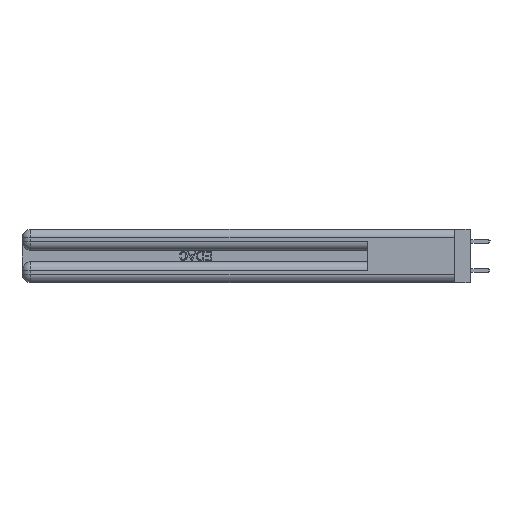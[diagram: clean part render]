
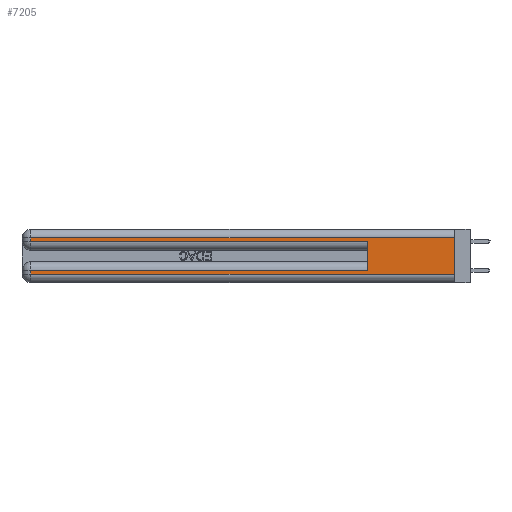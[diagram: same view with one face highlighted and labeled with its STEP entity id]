
A CAD part, left-side view. The second image highlights one B-rep face of the part: STEP entity #7205.
In plain terms, the highlighted planar face has unit normal (-1, 0, 0).
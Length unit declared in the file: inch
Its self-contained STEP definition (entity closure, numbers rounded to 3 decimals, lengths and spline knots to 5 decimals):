
#960 = EDGE_CURVE ( 'NONE', #34014, #14285, #3994, .T. ) ;
#1255 = CARTESIAN_POINT ( 'NONE',  ( 0., 0., 0.31 ) ) ;
#2277 = VECTOR ( 'NONE', #10742, 39.37008 ) ;
#3436 = CARTESIAN_POINT ( 'NONE',  ( 0., 0.6, 0.085 ) ) ;
#3994 = LINE ( 'NONE', #7187, #33371 ) ;
#4987 = ORIENTED_EDGE ( 'NONE', *, *, #38704, .T. ) ;
#5442 = LINE ( 'NONE', #36831, #28363 ) ;
#5456 = ORIENTED_EDGE ( 'NONE', *, *, #41916, .T. ) ;
#7187 = CARTESIAN_POINT ( 'NONE',  ( 0., 0.6, 0.145 ) ) ;
#7205 = ADVANCED_FACE ( 'NONE', ( #30709 ), #28962, .F. ) ;
#8068 = EDGE_CURVE ( 'NONE', #26083, #13559, #33846, .T. ) ;
#8346 = LINE ( 'NONE', #22822, #39291 ) ;
#10742 = DIRECTION ( 'NONE',  ( 0., 1., 0. ) ) ;
#10837 = VERTEX_POINT ( 'NONE', #41813 ) ;
#10854 = VECTOR ( 'NONE', #26650, 39.37008 ) ;
#11271 = CARTESIAN_POINT ( 'NONE',  ( 0., 0., 0.31 ) ) ;
#11644 = VECTOR ( 'NONE', #25696, 39.37008 ) ;
#11915 = LINE ( 'NONE', #27533, #2277 ) ;
#12110 = DIRECTION ( 'NONE',  ( 0., 0., -1. ) ) ;
#12236 = ORIENTED_EDGE ( 'NONE', *, *, #42745, .T. ) ;
#12563 = DIRECTION ( 'NONE',  ( 1., 0., 0. ) ) ;
#12837 = DIRECTION ( 'NONE',  ( 0., 0., -1. ) ) ;
#12926 = EDGE_LOOP ( 'NONE', ( #39824, #5456, #31135, #44123, #21703, #4987, #12236, #15629 ) ) ;
#13356 = VECTOR ( 'NONE', #18758, 39.37008 ) ;
#13559 = VERTEX_POINT ( 'NONE', #26681 ) ;
#14285 = VERTEX_POINT ( 'NONE', #33269 ) ;
#15629 = ORIENTED_EDGE ( 'NONE', *, *, #28323, .T. ) ;
#18758 = DIRECTION ( 'NONE',  ( 0., -1., 0. ) ) ;
#18905 = CARTESIAN_POINT ( 'NONE',  ( 0., 0., 0.06 ) ) ;
#20135 = EDGE_CURVE ( 'NONE', #41696, #10837, #23077, .T. ) ;
#20142 = EDGE_CURVE ( 'NONE', #10837, #14285, #5442, .T. ) ;
#20270 = CARTESIAN_POINT ( 'NONE',  ( 0., 2.94, 0.37 ) ) ;
#21246 = CARTESIAN_POINT ( 'NONE',  ( 0., 0., 0.37 ) ) ;
#21703 = ORIENTED_EDGE ( 'NONE', *, *, #960, .F. ) ;
#22822 = CARTESIAN_POINT ( 'NONE',  ( 0., 2.94, 0.37 ) ) ;
#23077 = LINE ( 'NONE', #20270, #10854 ) ;
#25696 = DIRECTION ( 'NONE',  ( 0., 1., 0. ) ) ;
#26083 = VERTEX_POINT ( 'NONE', #11271 ) ;
#26650 = DIRECTION ( 'NONE',  ( 0., 0., -1. ) ) ;
#26681 = CARTESIAN_POINT ( 'NONE',  ( 0., 0., 0.06 ) ) ;
#27533 = CARTESIAN_POINT ( 'NONE',  ( 0., 0., 0.085 ) ) ;
#28323 = EDGE_CURVE ( 'NONE', #43450, #13559, #40567, .T. ) ;
#28363 = VECTOR ( 'NONE', #40254, 39.37008 ) ;
#28826 = DIRECTION ( 'NONE',  ( 0., 0., -1. ) ) ;
#28962 = PLANE ( 'NONE',  #32299 ) ;
#29760 = CARTESIAN_POINT ( 'NONE',  ( 0., 2.94, 0.31 ) ) ;
#30709 = FACE_OUTER_BOUND ( 'NONE', #12926, .T. ) ;
#31049 = DIRECTION ( 'NONE',  ( 0., 0., 1. ) ) ;
#31135 = ORIENTED_EDGE ( 'NONE', *, *, #20135, .T. ) ;
#31692 = VECTOR ( 'NONE', #28826, 39.37008 ) ;
#32299 = AXIS2_PLACEMENT_3D ( 'NONE', #32560, #12563, #12110 ) ;
#32560 = CARTESIAN_POINT ( 'NONE',  ( 0., 0., 0.37 ) ) ;
#33269 = CARTESIAN_POINT ( 'NONE',  ( 0., 0.6, 0.285 ) ) ;
#33371 = VECTOR ( 'NONE', #31049, 39.37008 ) ;
#33846 = LINE ( 'NONE', #21246, #31692 ) ;
#34014 = VERTEX_POINT ( 'NONE', #3436 ) ;
#36831 = CARTESIAN_POINT ( 'NONE',  ( 0., 0., 0.285 ) ) ;
#38704 = EDGE_CURVE ( 'NONE', #34014, #42170, #11915, .T. ) ;
#38861 = LINE ( 'NONE', #1255, #11644 ) ;
#39291 = VECTOR ( 'NONE', #12837, 39.37008 ) ;
#39824 = ORIENTED_EDGE ( 'NONE', *, *, #8068, .F. ) ;
#39988 = CARTESIAN_POINT ( 'NONE',  ( 0., 2.94, 0.06 ) ) ;
#40174 = CARTESIAN_POINT ( 'NONE',  ( 0., 2.94, 0.085 ) ) ;
#40254 = DIRECTION ( 'NONE',  ( 0., -1., 0. ) ) ;
#40567 = LINE ( 'NONE', #18905, #13356 ) ;
#41696 = VERTEX_POINT ( 'NONE', #29760 ) ;
#41813 = CARTESIAN_POINT ( 'NONE',  ( 0., 2.94, 0.285 ) ) ;
#41916 = EDGE_CURVE ( 'NONE', #26083, #41696, #38861, .T. ) ;
#42170 = VERTEX_POINT ( 'NONE', #40174 ) ;
#42745 = EDGE_CURVE ( 'NONE', #42170, #43450, #8346, .T. ) ;
#43450 = VERTEX_POINT ( 'NONE', #39988 ) ;
#44123 = ORIENTED_EDGE ( 'NONE', *, *, #20142, .T. ) ;
